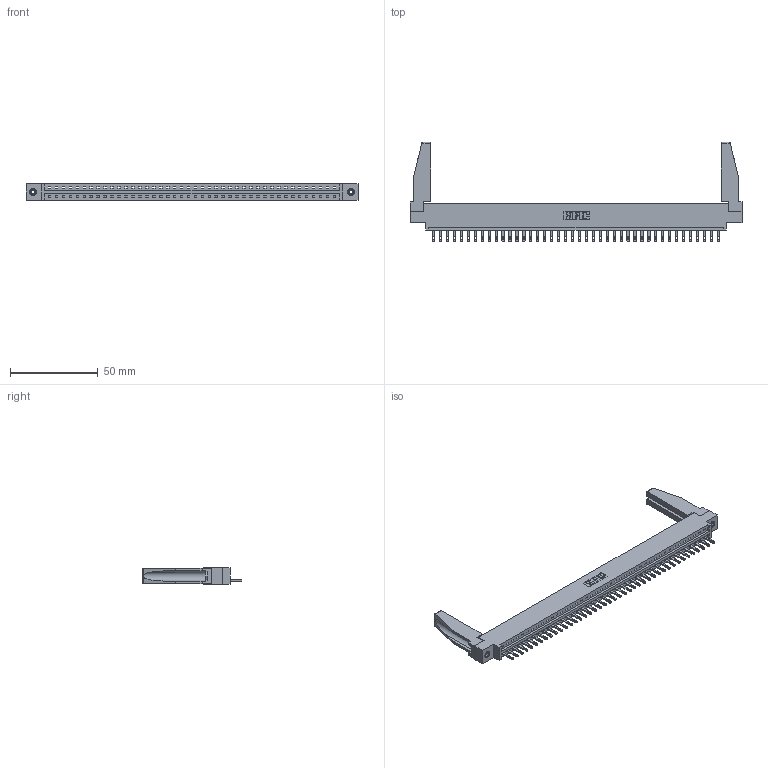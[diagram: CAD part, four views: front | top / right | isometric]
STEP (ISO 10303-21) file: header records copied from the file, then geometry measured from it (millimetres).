
FILE_DESCRIPTION (( 'STEP AP203' ), '1' );
FILE_NAME ('337-042-500-678.STEP', '2019-10-01T21:34:53', ( '' ), ( '' ), 'SwSTEP 2.0', 'SolidWorks 2016', '' );
FILE_SCHEMA (( 'CONFIG_CONTROL_DESIGN' ));
Length unit declared in the file: inch
Products named in the file (5): 337-042-500-678; 345-250-001_345-250-001-102; 345-292-001_345-293-100; 307-220-078; 337 Part_0.170 Offset - 0.156 Dia-TI
Assembly tree (47 placements, depth 2):
  337-042-500-678
    337 Part_0.170 Offset - 0.156 Dia-TI
    345-292-001_345-293-100  x42
    345-250-001_345-250-001-102  x2
    307-220-078  x2
Bounding box: 189.43 x 56.65 x 9.4 mm (x, y, z)
Volume: 23590.2 mm3; surface area: 24281.9 mm2
Topology: 47 solids, 47 shells, 2684 faces, 8213 edges, 5466 vertices
Faces by surface type: plane 1838, cylinder 830, cone 12, torus 4
Entity records: 33722 total; most frequent: CARTESIAN_POINT 5866, ORIENTED_EDGE 5800, DIRECTION 4948, EDGE_CURVE 2900, VECTOR 2730, LINE 2730, VERTEX_POINT 1928, AXIS2_PLACEMENT_3D 1109
